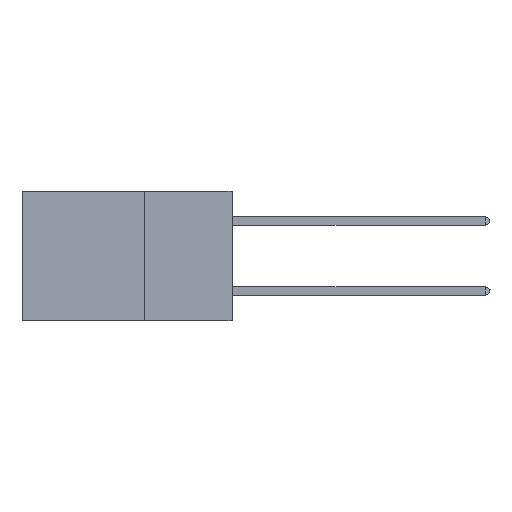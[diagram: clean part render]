
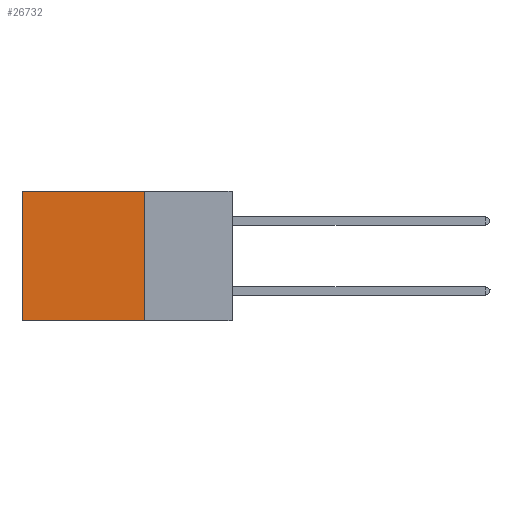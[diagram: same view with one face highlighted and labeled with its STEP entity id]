
A CAD part, left-side view. The second image highlights one B-rep face of the part: STEP entity #26732.
In plain terms, the highlighted planar face has unit normal (-1, 0, 0).
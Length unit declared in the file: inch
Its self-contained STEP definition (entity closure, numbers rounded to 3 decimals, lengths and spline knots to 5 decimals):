
#855 = VECTOR ( 'NONE', #2664, 39.37008 ) ;
#923 = VECTOR ( 'NONE', #15777, 39.37008 ) ;
#1004 = EDGE_LOOP ( 'NONE', ( #10864, #11061, #16639, #20142 ) ) ;
#2664 = DIRECTION ( 'NONE',  ( 0., 0., -1. ) ) ;
#4009 = VERTEX_POINT ( 'NONE', #11748 ) ;
#5521 = EDGE_CURVE ( 'NONE', #12962, #21534, #21700, .T. ) ;
#5891 = DIRECTION ( 'NONE',  ( 0., 1., 0. ) ) ;
#6265 = CARTESIAN_POINT ( 'NONE',  ( 0.2875, 0.25, -0.37 ) ) ;
#6589 = DIRECTION ( 'NONE',  ( 0., 0., -1. ) ) ;
#7206 = CARTESIAN_POINT ( 'NONE',  ( 0.2875, 0.6, 0. ) ) ;
#9992 = VECTOR ( 'NONE', #15743, 39.37008 ) ;
#10864 = ORIENTED_EDGE ( 'NONE', *, *, #5521, .T. ) ;
#11061 = ORIENTED_EDGE ( 'NONE', *, *, #27400, .F. ) ;
#11335 = LINE ( 'NONE', #22152, #9992 ) ;
#11653 = CARTESIAN_POINT ( 'NONE',  ( 0.2875, 0.25, -0.37 ) ) ;
#11748 = CARTESIAN_POINT ( 'NONE',  ( 0.2875, 0.25, 0. ) ) ;
#11752 = PLANE ( 'NONE',  #24906 ) ;
#12522 = VECTOR ( 'NONE', #5891, 39.37008 ) ;
#12962 = VERTEX_POINT ( 'NONE', #17654 ) ;
#13645 = LINE ( 'NONE', #11653, #923 ) ;
#13933 = EDGE_CURVE ( 'NONE', #4009, #24513, #11335, .T. ) ;
#15743 = DIRECTION ( 'NONE',  ( 0., 0., -1. ) ) ;
#15777 = DIRECTION ( 'NONE',  ( 0., 1., 0. ) ) ;
#16639 = ORIENTED_EDGE ( 'NONE', *, *, #13933, .F. ) ;
#17654 = CARTESIAN_POINT ( 'NONE',  ( 0.2875, 0.6, 0. ) ) ;
#18812 = CARTESIAN_POINT ( 'NONE',  ( 0.2875, 0.25, 0. ) ) ;
#19019 = CARTESIAN_POINT ( 'NONE',  ( 0.2875, 0.6, -0.37 ) ) ;
#20142 = ORIENTED_EDGE ( 'NONE', *, *, #23715, .T. ) ;
#20433 = CARTESIAN_POINT ( 'NONE',  ( 0.2875, 0.25, 0. ) ) ;
#21534 = VERTEX_POINT ( 'NONE', #19019 ) ;
#21700 = LINE ( 'NONE', #7206, #855 ) ;
#22152 = CARTESIAN_POINT ( 'NONE',  ( 0.2875, 0.25, 0. ) ) ;
#22973 = FACE_OUTER_BOUND ( 'NONE', #1004, .T. ) ;
#23715 = EDGE_CURVE ( 'NONE', #4009, #12962, #25613, .T. ) ;
#24513 = VERTEX_POINT ( 'NONE', #6265 ) ;
#24906 = AXIS2_PLACEMENT_3D ( 'NONE', #20433, #25898, #6589 ) ;
#25613 = LINE ( 'NONE', #18812, #12522 ) ;
#25898 = DIRECTION ( 'NONE',  ( 1., 0., 0. ) ) ;
#26732 = ADVANCED_FACE ( 'NONE', ( #22973 ), #11752, .F. ) ;
#27400 = EDGE_CURVE ( 'NONE', #24513, #21534, #13645, .T. ) ;
